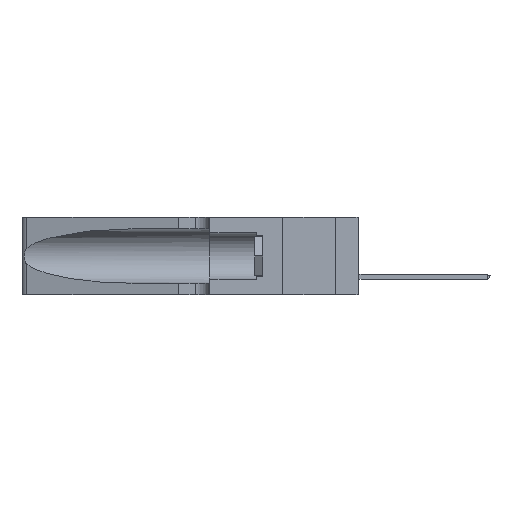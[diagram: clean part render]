
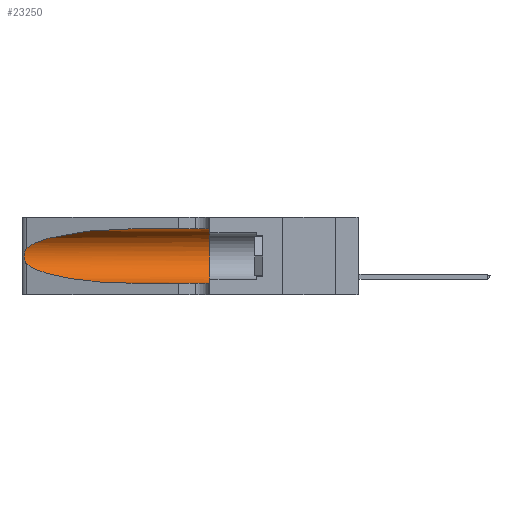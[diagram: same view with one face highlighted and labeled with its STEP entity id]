
A CAD part, left-side view. The second image highlights one B-rep face of the part: STEP entity #23250.
In plain terms, the highlighted cylindrical face has radius 3.308 mm (diameter 6.617 mm), a partial arc.
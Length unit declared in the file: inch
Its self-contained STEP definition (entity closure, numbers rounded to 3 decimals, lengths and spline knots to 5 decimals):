
#1315 = CARTESIAN_POINT ( 'NONE',  ( 0.25639, 1.23186, 0.15144 ) ) ;
#1733 = CARTESIAN_POINT ( 'NONE',  ( 0.25555, 1.22994, 0.2215 ) ) ;
#2507 = LINE ( 'NONE', #33987, #35702 ) ;
#2993 = ORIENTED_EDGE ( 'NONE', *, *, #28227, .T. ) ;
#3790 = EDGE_CURVE ( 'NONE', #21313, #5869, #22890, .T. ) ;
#4333 = VERTEX_POINT ( 'NONE', #19201 ) ;
#4553 = CARTESIAN_POINT ( 'NONE',  ( 0.26075, 1.23896, 0.178 ) ) ;
#5500 = EDGE_CURVE ( 'NONE', #5996, #5869, #34976, .T. ) ;
#5869 = VERTEX_POINT ( 'NONE', #20502 ) ;
#5996 = VERTEX_POINT ( 'NONE', #31505 ) ;
#7555 = ORIENTED_EDGE ( 'NONE', *, *, #5500, .F. ) ;
#7670 = CARTESIAN_POINT ( 'NONE',  ( 0.25787, 1.23484, 0.2124 ) ) ;
#8044 = CARTESIAN_POINT ( 'NONE',  ( 0.25487, 1.22718, 0.14631 ) ) ;
#8457 = CARTESIAN_POINT ( 'NONE',  ( 0.18966, 0.96281, 0.31525 ) ) ;
#10250 = EDGE_CURVE ( 'NONE', #4333, #36287, #22602, .T. ) ;
#10736 = EDGE_CURVE ( 'NONE', #36287, #18134, #17351, .T. ) ;
#10877 = CARTESIAN_POINT ( 'NONE',  ( 0.1305, 0.72297, 0.05475 ) ) ;
#10942 = CARTESIAN_POINT ( 'NONE',  ( 0.25487, 1.22718, 0.14631 ) ) ;
#11775 = ORIENTED_EDGE ( 'NONE', *, *, #3790, .T. ) ;
#12818 =( BOUNDED_CURVE ( )  B_SPLINE_CURVE ( 3, ( #8044, #22905, #17523, #37885 ),
 .UNSPECIFIED., .F., .F. ) 
 B_SPLINE_CURVE_WITH_KNOTS ( ( 4, 4 ),
 ( 3.44316, 4.71239 ),
 .UNSPECIFIED. ) 
 CURVE ( )  GEOMETRIC_REPRESENTATION_ITEM ( )  RATIONAL_B_SPLINE_CURVE ( ( 1., 0.87, 0.87, 1. ) ) 
 REPRESENTATION_ITEM ( '' )  );
#13255 = CARTESIAN_POINT ( 'NONE',  ( 0.1305, 0.35, 0.185 ) ) ;
#13592 = CARTESIAN_POINT ( 'NONE',  ( 0.25639, 1.23184, 0.21858 ) ) ;
#14045 = AXIS2_PLACEMENT_3D ( 'NONE', #30413, #33234, #33637 ) ;
#15031 = FACE_OUTER_BOUND ( 'NONE', #27425, .T. ) ;
#16018 = CARTESIAN_POINT ( 'NONE',  ( 0.25555, 1.22993, 0.14849 ) ) ;
#16220 = DIRECTION ( 'NONE',  ( 0., 0., 1. ) ) ;
#17351 = B_SPLINE_CURVE_WITH_KNOTS ( 'NONE', 3,
 ( #25277, #1733, #13592, #7670, #33996, #36810, #22134, #4553, #19269, #25014, #25418, #1315, #16018, #22275 ),
 .UNSPECIFIED., .F., .F.,
 ( 4, 2, 2, 2, 2, 2, 4 ),
 ( 0., 0.00027, 0.00053, 0.00107, 0.0016, 0.00187, 0.00214 ),
 .UNSPECIFIED. ) ;
#17523 = CARTESIAN_POINT ( 'NONE',  ( 0.18966, 0.96281, 0.05475 ) ) ;
#18134 = VERTEX_POINT ( 'NONE', #10942 ) ;
#18171 = CARTESIAN_POINT ( 'NONE',  ( 0.2373, 1.15595, 0.28018 ) ) ;
#18597 = AXIS2_PLACEMENT_3D ( 'NONE', #13255, #32881, #16220 ) ;
#19201 = CARTESIAN_POINT ( 'NONE',  ( 0.1305, 0.72297, 0.31525 ) ) ;
#19269 = CARTESIAN_POINT ( 'NONE',  ( 0.26017, 1.23833, 0.17102 ) ) ;
#19283 = ORIENTED_EDGE ( 'NONE', *, *, #25195, .F. ) ;
#19794 = DIRECTION ( 'NONE',  ( 0., -1., 0. ) ) ;
#20502 = CARTESIAN_POINT ( 'NONE',  ( 0.1305, 0.35, 0.05475 ) ) ;
#21313 = VERTEX_POINT ( 'NONE', #10877 ) ;
#21427 = VECTOR ( 'NONE', #25534, 39.37008 ) ;
#21994 = CYLINDRICAL_SURFACE ( 'NONE', #14045, 0.13025 ) ;
#22134 = CARTESIAN_POINT ( 'NONE',  ( 0.26075, 1.23896, 0.19203 ) ) ;
#22275 = CARTESIAN_POINT ( 'NONE',  ( 0.25487, 1.22718, 0.14631 ) ) ;
#22602 =( BOUNDED_CURVE ( )  B_SPLINE_CURVE ( 3, ( #37748, #8457, #18171, #29835 ),
 .UNSPECIFIED., .F., .T. ) 
 B_SPLINE_CURVE_WITH_KNOTS ( ( 4, 4 ),
 ( 1.5708, 2.84003 ),
 .UNSPECIFIED. ) 
 CURVE ( )  GEOMETRIC_REPRESENTATION_ITEM ( )  RATIONAL_B_SPLINE_CURVE ( ( 1., 0.87, 0.87, 1. ) ) 
 REPRESENTATION_ITEM ( '' )  );
#22890 = LINE ( 'NONE', #31271, #21427 ) ;
#22905 = CARTESIAN_POINT ( 'NONE',  ( 0.2373, 1.15595, 0.08982 ) ) ;
#23250 = ADVANCED_FACE ( 'NONE', ( #15031 ), #21994, .F. ) ;
#25014 = CARTESIAN_POINT ( 'NONE',  ( 0.25856, 1.23593, 0.16098 ) ) ;
#25195 = EDGE_CURVE ( 'NONE', #4333, #5996, #2507, .T. ) ;
#25277 = CARTESIAN_POINT ( 'NONE',  ( 0.25487, 1.22718, 0.22369 ) ) ;
#25418 = CARTESIAN_POINT ( 'NONE',  ( 0.25789, 1.23486, 0.15765 ) ) ;
#25534 = DIRECTION ( 'NONE',  ( 0., -1., 0. ) ) ;
#26710 = ORIENTED_EDGE ( 'NONE', *, *, #10736, .T. ) ;
#27425 = EDGE_LOOP ( 'NONE', ( #33080, #26710, #2993, #11775, #7555, #19283 ) ) ;
#28227 = EDGE_CURVE ( 'NONE', #18134, #21313, #12818, .T. ) ;
#29835 = CARTESIAN_POINT ( 'NONE',  ( 0.25487, 1.22718, 0.22369 ) ) ;
#30413 = CARTESIAN_POINT ( 'NONE',  ( 0.1305, 1.61858, 0.185 ) ) ;
#31271 = CARTESIAN_POINT ( 'NONE',  ( 0.1305, 1.61858, 0.05475 ) ) ;
#31505 = CARTESIAN_POINT ( 'NONE',  ( 0.1305, 0.35, 0.31525 ) ) ;
#32881 = DIRECTION ( 'NONE',  ( 0., 1., 0. ) ) ;
#33080 = ORIENTED_EDGE ( 'NONE', *, *, #10250, .T. ) ;
#33234 = DIRECTION ( 'NONE',  ( 0., -1., 0. ) ) ;
#33637 = DIRECTION ( 'NONE',  ( 0., 0., -1. ) ) ;
#33788 = CARTESIAN_POINT ( 'NONE',  ( 0.25487, 1.22718, 0.22369 ) ) ;
#33987 = CARTESIAN_POINT ( 'NONE',  ( 0.1305, 1.61858, 0.31525 ) ) ;
#33996 = CARTESIAN_POINT ( 'NONE',  ( 0.25854, 1.2359, 0.20912 ) ) ;
#34976 = CIRCLE ( 'NONE', #18597, 0.13025 ) ;
#35702 = VECTOR ( 'NONE', #19794, 39.37008 ) ;
#36287 = VERTEX_POINT ( 'NONE', #33788 ) ;
#36810 = CARTESIAN_POINT ( 'NONE',  ( 0.26018, 1.23835, 0.19895 ) ) ;
#37748 = CARTESIAN_POINT ( 'NONE',  ( 0.1305, 0.72297, 0.31525 ) ) ;
#37885 = CARTESIAN_POINT ( 'NONE',  ( 0.1305, 0.72297, 0.05475 ) ) ;
